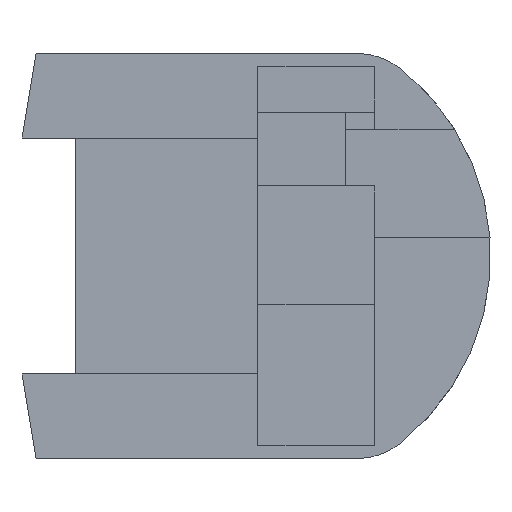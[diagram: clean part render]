
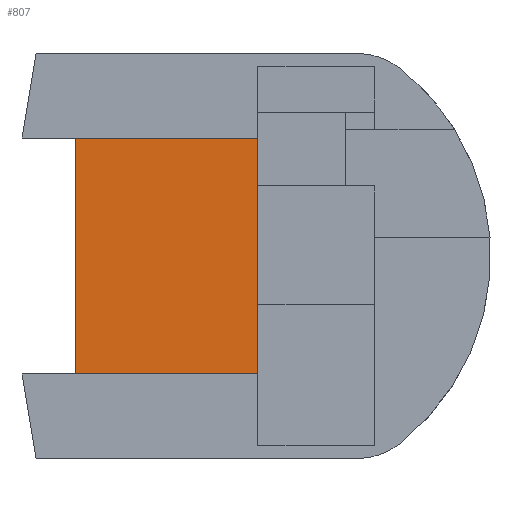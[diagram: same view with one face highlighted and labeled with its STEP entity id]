
A CAD part, front view. The second image highlights one B-rep face of the part: STEP entity #807.
In plain terms, the highlighted planar face has unit normal (0, -1, 0).
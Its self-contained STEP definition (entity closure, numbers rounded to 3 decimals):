
#6 = PLANE ( 'NONE',  #1122 ) ;
#21 = CARTESIAN_POINT ( 'NONE',  ( -77.303, 10.236, -4.934 ) ) ;
#153 = EDGE_CURVE ( 'NONE', #1333, #884, #2278, .T. ) ;
#162 = LINE ( 'NONE', #21, #663 ) ;
#249 = CARTESIAN_POINT ( 'NONE',  ( -75.074, 10.236, 4.934 ) ) ;
#250 = CARTESIAN_POINT ( 'NONE',  ( -67.443, 10.236, 4.934 ) ) ;
#288 = ORIENTED_EDGE ( 'NONE', *, *, #153, .F. ) ;
#354 = EDGE_CURVE ( 'NONE', #2373, #1333, #162, .T. ) ;
#358 = CARTESIAN_POINT ( 'NONE',  ( -67.443, 10.236, 4.934 ) ) ;
#432 = EDGE_CURVE ( 'NONE', #884, #1809, #1289, .T. ) ;
#546 = ORIENTED_EDGE ( 'NONE', *, *, #432, .F. ) ;
#645 = DIRECTION ( 'NONE',  ( 0., 1., 0. ) ) ;
#663 = VECTOR ( 'NONE', #1379, 1000. ) ;
#691 = FACE_OUTER_BOUND ( 'NONE', #1807, .T. ) ;
#697 = DIRECTION ( 'NONE',  ( 1., 0., 0. ) ) ;
#807 = ADVANCED_FACE ( 'NONE', ( #691 ), #6, .F. ) ;
#884 = VERTEX_POINT ( 'NONE', #249 ) ;
#968 = LINE ( 'NONE', #1953, #2487 ) ;
#1089 = EDGE_CURVE ( 'NONE', #1809, #2373, #968, .T. ) ;
#1122 = AXIS2_PLACEMENT_3D ( 'NONE', #1853, #645, #2045 ) ;
#1237 = ORIENTED_EDGE ( 'NONE', *, *, #354, .F. ) ;
#1289 = LINE ( 'NONE', #250, #1362 ) ;
#1333 = VERTEX_POINT ( 'NONE', #1918 ) ;
#1362 = VECTOR ( 'NONE', #697, 1000. ) ;
#1374 = DIRECTION ( 'NONE',  ( 0., 0., 1. ) ) ;
#1379 = DIRECTION ( 'NONE',  ( -1., 0., 0. ) ) ;
#1656 = CARTESIAN_POINT ( 'NONE',  ( -75.074, 10.236, -3.096 ) ) ;
#1772 = VECTOR ( 'NONE', #1374, 1000. ) ;
#1807 = EDGE_LOOP ( 'NONE', ( #288, #1237, #1967, #546 ) ) ;
#1809 = VERTEX_POINT ( 'NONE', #358 ) ;
#1853 = CARTESIAN_POINT ( 'NONE',  ( -72.494, 10.236, 0. ) ) ;
#1918 = CARTESIAN_POINT ( 'NONE',  ( -75.074, 10.236, -4.934 ) ) ;
#1953 = CARTESIAN_POINT ( 'NONE',  ( -67.443, 10.236, -7.925 ) ) ;
#1967 = ORIENTED_EDGE ( 'NONE', *, *, #1089, .F. ) ;
#2045 = DIRECTION ( 'NONE',  ( 0., 0., 1. ) ) ;
#2148 = DIRECTION ( 'NONE',  ( 0., 0., -1. ) ) ;
#2278 = LINE ( 'NONE', #1656, #1772 ) ;
#2317 = CARTESIAN_POINT ( 'NONE',  ( -67.443, 10.236, -4.934 ) ) ;
#2373 = VERTEX_POINT ( 'NONE', #2317 ) ;
#2487 = VECTOR ( 'NONE', #2148, 1000. ) ;
